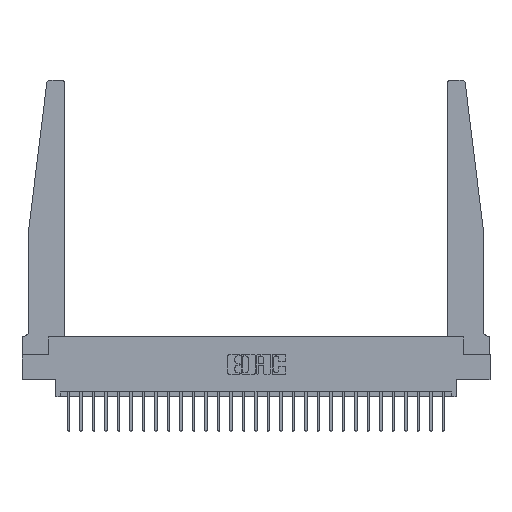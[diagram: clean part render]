
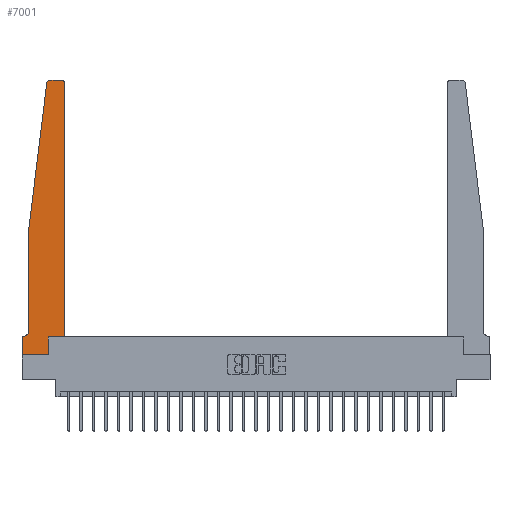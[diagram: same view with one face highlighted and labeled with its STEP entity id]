
A CAD part, top view. The second image highlights one B-rep face of the part: STEP entity #7001.
In plain terms, the highlighted planar face has unit normal (0, 0, 1).
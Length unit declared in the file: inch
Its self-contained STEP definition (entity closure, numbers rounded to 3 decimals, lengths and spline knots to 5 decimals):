
#190 = CARTESIAN_POINT ( 'NONE',  ( 0., 0., 0.37 ) ) ;
#794 = AXIS2_PLACEMENT_3D ( 'NONE', #13180, #21118, #23448 ) ;
#800 = EDGE_CURVE ( 'NONE', #6275, #19118, #6708, .T. ) ;
#1061 = EDGE_CURVE ( 'NONE', #21089, #3137, #13941, .T. ) ;
#1241 = ORIENTED_EDGE ( 'NONE', *, *, #9107, .T. ) ;
#1794 = CARTESIAN_POINT ( 'NONE',  ( 0., 0.1875, 0.37 ) ) ;
#2000 = ORIENTED_EDGE ( 'NONE', *, *, #24614, .T. ) ;
#2084 = DIRECTION ( 'NONE',  ( -1., 0., 0. ) ) ;
#2091 = EDGE_CURVE ( 'NONE', #5437, #16684, #26970, .T. ) ;
#2379 = LINE ( 'NONE', #4848, #12312 ) ;
#3137 = VERTEX_POINT ( 'NONE', #190 ) ;
#3515 = AXIS2_PLACEMENT_3D ( 'NONE', #4336, #8296, #12958 ) ;
#3807 = DIRECTION ( 'NONE',  ( 0., -1., 0. ) ) ;
#3872 = CARTESIAN_POINT ( 'NONE',  ( 0.2605, 0.18, 0.37 ) ) ;
#4245 = FACE_OUTER_BOUND ( 'NONE', #20749, .T. ) ;
#4301 = CARTESIAN_POINT ( 'NONE',  ( 0.395, 2.75, 0.37 ) ) ;
#4336 = CARTESIAN_POINT ( 'NONE',  ( 0.27653, 2.72, 0.37 ) ) ;
#4370 = CIRCLE ( 'NONE', #3515, 0.03 ) ;
#4426 = CARTESIAN_POINT ( 'NONE',  ( 0.25, 2.75, 0.37 ) ) ;
#4721 = CARTESIAN_POINT ( 'NONE',  ( 0.24675, 2.72367, 0.37 ) ) ;
#4848 = CARTESIAN_POINT ( 'NONE',  ( 0., 0., 0.37 ) ) ;
#5430 = VERTEX_POINT ( 'NONE', #13048 ) ;
#5437 = VERTEX_POINT ( 'NONE', #19844 ) ;
#5455 = DIRECTION ( 'NONE',  ( 1., 0., 0. ) ) ;
#5517 = CARTESIAN_POINT ( 'NONE',  ( 0.065, 1.25, 0.37 ) ) ;
#5592 = CARTESIAN_POINT ( 'NONE',  ( 0.425, 0.18, 0.37 ) ) ;
#5603 = VECTOR ( 'NONE', #2084, 39.37008 ) ;
#6275 = VERTEX_POINT ( 'NONE', #4721 ) ;
#6278 = ORIENTED_EDGE ( 'NONE', *, *, #6377, .T. ) ;
#6324 = LINE ( 'NONE', #4426, #5603 ) ;
#6377 = EDGE_CURVE ( 'NONE', #19118, #23566, #17987, .T. ) ;
#6419 = CARTESIAN_POINT ( 'NONE',  ( 0.425, 0.18, 0.37 ) ) ;
#6549 = VECTOR ( 'NONE', #16971, 39.37008 ) ;
#6708 = LINE ( 'NONE', #10827, #6549 ) ;
#7001 = ADVANCED_FACE ( 'NONE', ( #4245 ), #20289, .T. ) ;
#7016 = VECTOR ( 'NONE', #22825, 39.37008 ) ;
#8117 = VECTOR ( 'NONE', #13313, 39.37008 ) ;
#8296 = DIRECTION ( 'NONE',  ( 0., 0., 1. ) ) ;
#9107 = EDGE_CURVE ( 'NONE', #12937, #6275, #4370, .T. ) ;
#9824 = CARTESIAN_POINT ( 'NONE',  ( 0.015, 0.1875, 0.37 ) ) ;
#9987 = ORIENTED_EDGE ( 'NONE', *, *, #26395, .T. ) ;
#10039 = DIRECTION ( 'NONE',  ( 0., 1., 0. ) ) ;
#10050 = VECTOR ( 'NONE', #5455, 39.37008 ) ;
#10155 = DIRECTION ( 'NONE',  ( 1., 0., 0. ) ) ;
#10827 = CARTESIAN_POINT ( 'NONE',  ( 0.065, 1.25, 0.37 ) ) ;
#11809 = VECTOR ( 'NONE', #3807, 39.37008 ) ;
#12022 = CARTESIAN_POINT ( 'NONE',  ( 0.065, 0.2375, 0.37 ) ) ;
#12312 = VECTOR ( 'NONE', #19076, 39.37008 ) ;
#12658 = CARTESIAN_POINT ( 'NONE',  ( 0.27653, 2.75, 0.37 ) ) ;
#12865 = VERTEX_POINT ( 'NONE', #4301 ) ;
#12928 = ORIENTED_EDGE ( 'NONE', *, *, #21141, .T. ) ;
#12937 = VERTEX_POINT ( 'NONE', #12658 ) ;
#12958 = DIRECTION ( 'NONE',  ( 1., 0., 0. ) ) ;
#13048 = CARTESIAN_POINT ( 'NONE',  ( 0.425, 2.72, 0.37 ) ) ;
#13180 = CARTESIAN_POINT ( 'NONE',  ( 0.395, 2.72, 0.37 ) ) ;
#13313 = DIRECTION ( 'NONE',  ( 0., 1., 0. ) ) ;
#13431 = VECTOR ( 'NONE', #10039, 39.37008 ) ;
#13525 = VERTEX_POINT ( 'NONE', #17402 ) ;
#13744 = DIRECTION ( 'NONE',  ( 0., -1., 0. ) ) ;
#13941 = LINE ( 'NONE', #18175, #11809 ) ;
#14046 = DIRECTION ( 'NONE',  ( 0., 0., -1. ) ) ;
#15605 = LINE ( 'NONE', #16786, #7016 ) ;
#16131 = CIRCLE ( 'NONE', #20517, 0.05 ) ;
#16227 = DIRECTION ( 'NONE',  ( -1., 0., 0. ) ) ;
#16684 = VERTEX_POINT ( 'NONE', #6419 ) ;
#16728 = ORIENTED_EDGE ( 'NONE', *, *, #800, .T. ) ;
#16786 = CARTESIAN_POINT ( 'NONE',  ( 0.065, 0.1875, 0.37 ) ) ;
#16958 = EDGE_CURVE ( 'NONE', #22243, #21089, #15605, .T. ) ;
#16971 = DIRECTION ( 'NONE',  ( -0.122, -0.992, 0. ) ) ;
#17285 = CARTESIAN_POINT ( 'NONE',  ( 0., 0.1875, 0.37 ) ) ;
#17402 = CARTESIAN_POINT ( 'NONE',  ( 0.2605, 0., 0.37 ) ) ;
#17608 = CARTESIAN_POINT ( 'NONE',  ( 0.015, 0.2375, 0.37 ) ) ;
#17678 = LINE ( 'NONE', #17810, #8117 ) ;
#17810 = CARTESIAN_POINT ( 'NONE',  ( 0.425, 0.18, 0.37 ) ) ;
#17987 = LINE ( 'NONE', #24027, #22774 ) ;
#18175 = CARTESIAN_POINT ( 'NONE',  ( 0., 0., 0.37 ) ) ;
#18360 = DIRECTION ( 'NONE',  ( 0., 0., 1. ) ) ;
#18784 = LINE ( 'NONE', #3872, #13431 ) ;
#19076 = DIRECTION ( 'NONE',  ( 1., 0., 0. ) ) ;
#19108 = ORIENTED_EDGE ( 'NONE', *, *, #16958, .T. ) ;
#19118 = VERTEX_POINT ( 'NONE', #5517 ) ;
#19378 = ORIENTED_EDGE ( 'NONE', *, *, #24004, .T. ) ;
#19844 = CARTESIAN_POINT ( 'NONE',  ( 0.2605, 0.18, 0.37 ) ) ;
#20289 = PLANE ( 'NONE',  #24579 ) ;
#20517 = AXIS2_PLACEMENT_3D ( 'NONE', #17608, #14046, #16227 ) ;
#20749 = EDGE_LOOP ( 'NONE', ( #2000, #1241, #16728, #6278, #19378, #19108, #20870, #12928, #9987, #22711, #22514, #26832 ) ) ;
#20870 = ORIENTED_EDGE ( 'NONE', *, *, #1061, .T. ) ;
#21089 = VERTEX_POINT ( 'NONE', #17285 ) ;
#21118 = DIRECTION ( 'NONE',  ( 0., 0., 1. ) ) ;
#21141 = EDGE_CURVE ( 'NONE', #3137, #13525, #2379, .T. ) ;
#22243 = VERTEX_POINT ( 'NONE', #9824 ) ;
#22514 = ORIENTED_EDGE ( 'NONE', *, *, #25275, .T. ) ;
#22711 = ORIENTED_EDGE ( 'NONE', *, *, #2091, .T. ) ;
#22774 = VECTOR ( 'NONE', #13744, 39.37008 ) ;
#22825 = DIRECTION ( 'NONE',  ( -1., 0., 0. ) ) ;
#22870 = EDGE_CURVE ( 'NONE', #5430, #12865, #23540, .T. ) ;
#23448 = DIRECTION ( 'NONE',  ( 1., 0., 0. ) ) ;
#23540 = CIRCLE ( 'NONE', #794, 0.03 ) ;
#23566 = VERTEX_POINT ( 'NONE', #12022 ) ;
#24004 = EDGE_CURVE ( 'NONE', #23566, #22243, #16131, .T. ) ;
#24027 = CARTESIAN_POINT ( 'NONE',  ( 0.065, 1.25, 0.37 ) ) ;
#24579 = AXIS2_PLACEMENT_3D ( 'NONE', #1794, #18360, #10155 ) ;
#24614 = EDGE_CURVE ( 'NONE', #12865, #12937, #6324, .T. ) ;
#25275 = EDGE_CURVE ( 'NONE', #16684, #5430, #17678, .T. ) ;
#26395 = EDGE_CURVE ( 'NONE', #13525, #5437, #18784, .T. ) ;
#26832 = ORIENTED_EDGE ( 'NONE', *, *, #22870, .T. ) ;
#26970 = LINE ( 'NONE', #5592, #10050 ) ;
